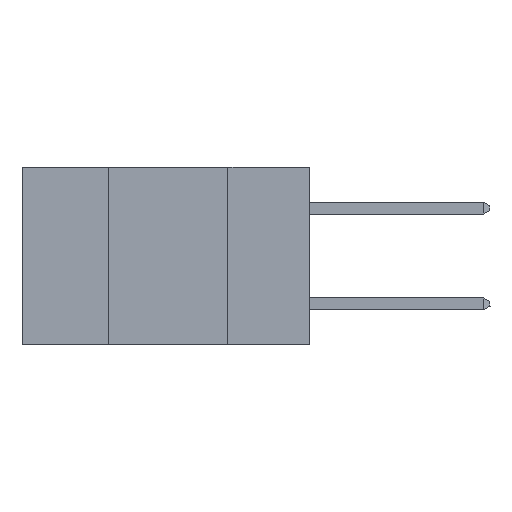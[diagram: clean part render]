
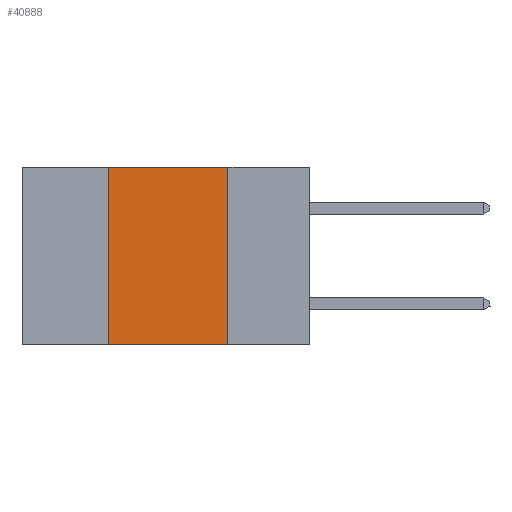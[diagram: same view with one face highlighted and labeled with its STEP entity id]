
A CAD part, left-side view. The second image highlights one B-rep face of the part: STEP entity #40888.
In plain terms, the highlighted planar face has unit normal (-1, 0, 0).
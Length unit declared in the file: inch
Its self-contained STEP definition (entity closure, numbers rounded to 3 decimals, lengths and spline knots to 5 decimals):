
#51 = VERTEX_POINT ( 'NONE', #33280 ) ;
#1088 = VERTEX_POINT ( 'NONE', #37481 ) ;
#1476 = VECTOR ( 'NONE', #19421, 39.37008 ) ;
#2273 = VERTEX_POINT ( 'NONE', #15534 ) ;
#4084 = CARTESIAN_POINT ( 'NONE',  ( 0., 0.42, 0. ) ) ;
#6936 = EDGE_CURVE ( 'NONE', #51, #2273, #30107, .T. ) ;
#7318 = VECTOR ( 'NONE', #7622, 39.37008 ) ;
#7622 = DIRECTION ( 'NONE',  ( 0., 0., 1. ) ) ;
#9983 = EDGE_CURVE ( 'NONE', #51, #1088, #26003, .T. ) ;
#10859 = ORIENTED_EDGE ( 'NONE', *, *, #9983, .F. ) ;
#11867 = DIRECTION ( 'NONE',  ( 1., 0., 0. ) ) ;
#15534 = CARTESIAN_POINT ( 'NONE',  ( 0., 0.17, -0.37 ) ) ;
#17584 = CARTESIAN_POINT ( 'NONE',  ( 0., 0.17, 0. ) ) ;
#17585 = CARTESIAN_POINT ( 'NONE',  ( 0., 0.17, 0. ) ) ;
#18782 = LINE ( 'NONE', #17585, #28047 ) ;
#18785 = EDGE_LOOP ( 'NONE', ( #23482, #29513, #10859, #26224 ) ) ;
#19421 = DIRECTION ( 'NONE',  ( 0., -1., 0. ) ) ;
#20631 = EDGE_CURVE ( 'NONE', #37391, #2273, #18782, .T. ) ;
#20826 = VECTOR ( 'NONE', #28506, 39.37008 ) ;
#21030 = FACE_OUTER_BOUND ( 'NONE', #18785, .T. ) ;
#23246 = EDGE_CURVE ( 'NONE', #1088, #37391, #29509, .T. ) ;
#23482 = ORIENTED_EDGE ( 'NONE', *, *, #20631, .F. ) ;
#24990 = CARTESIAN_POINT ( 'NONE',  ( 0., 0.6, -0.37 ) ) ;
#26003 = LINE ( 'NONE', #4084, #7318 ) ;
#26224 = ORIENTED_EDGE ( 'NONE', *, *, #6936, .T. ) ;
#28047 = VECTOR ( 'NONE', #41991, 39.37008 ) ;
#28506 = DIRECTION ( 'NONE',  ( 0., -1., 0. ) ) ;
#29334 = PLANE ( 'NONE',  #32807 ) ;
#29509 = LINE ( 'NONE', #40289, #1476 ) ;
#29513 = ORIENTED_EDGE ( 'NONE', *, *, #23246, .F. ) ;
#30107 = LINE ( 'NONE', #24990, #20826 ) ;
#32807 = AXIS2_PLACEMENT_3D ( 'NONE', #32830, #11867, #36358 ) ;
#32830 = CARTESIAN_POINT ( 'NONE',  ( 0., 0.6, 0. ) ) ;
#33280 = CARTESIAN_POINT ( 'NONE',  ( 0., 0.42, -0.37 ) ) ;
#36358 = DIRECTION ( 'NONE',  ( 0., 0., -1. ) ) ;
#37391 = VERTEX_POINT ( 'NONE', #17584 ) ;
#37481 = CARTESIAN_POINT ( 'NONE',  ( 0., 0.42, 0. ) ) ;
#40289 = CARTESIAN_POINT ( 'NONE',  ( 0., 0.6, 0. ) ) ;
#40888 = ADVANCED_FACE ( 'NONE', ( #21030 ), #29334, .F. ) ;
#41991 = DIRECTION ( 'NONE',  ( 0., 0., -1. ) ) ;
